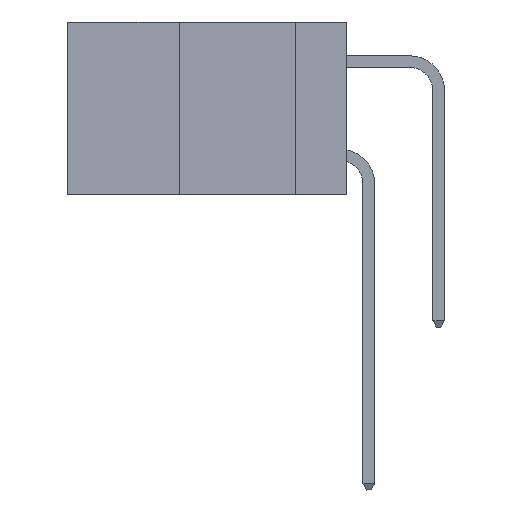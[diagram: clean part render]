
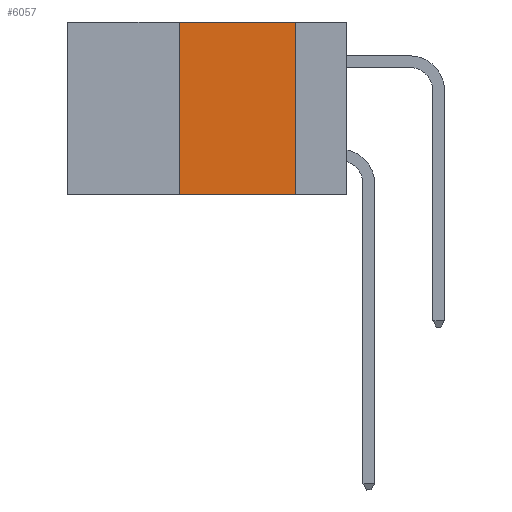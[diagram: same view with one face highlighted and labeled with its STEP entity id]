
A CAD part, left-side view. The second image highlights one B-rep face of the part: STEP entity #6057.
In plain terms, the highlighted planar face has unit normal (-1, 0, 0).
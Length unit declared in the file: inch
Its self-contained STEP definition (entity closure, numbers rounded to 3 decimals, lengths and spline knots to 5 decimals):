
#1659 = CARTESIAN_POINT ( 'NONE',  ( 0., 0.36, 0. ) ) ;
#2064 = AXIS2_PLACEMENT_3D ( 'NONE', #19146, #19528, #15060 ) ;
#2625 = VECTOR ( 'NONE', #18757, 39.37008 ) ;
#2629 = EDGE_CURVE ( 'NONE', #13762, #18556, #5952, .T. ) ;
#4824 = VECTOR ( 'NONE', #17352, 39.37008 ) ;
#4913 = CARTESIAN_POINT ( 'NONE',  ( 0., 0.36, -0.37 ) ) ;
#5952 = LINE ( 'NONE', #14203, #7526 ) ;
#6057 = ADVANCED_FACE ( 'NONE', ( #25244 ), #11332, .F. ) ;
#6169 = LINE ( 'NONE', #12888, #2625 ) ;
#7526 = VECTOR ( 'NONE', #21658, 39.37008 ) ;
#8325 = VERTEX_POINT ( 'NONE', #21366 ) ;
#9837 = EDGE_CURVE ( 'NONE', #8325, #16866, #6169, .T. ) ;
#10703 = CARTESIAN_POINT ( 'NONE',  ( 0., 0.11, 0. ) ) ;
#11332 = PLANE ( 'NONE',  #2064 ) ;
#12888 = CARTESIAN_POINT ( 'NONE',  ( 0., 0.6, 0. ) ) ;
#13762 = VERTEX_POINT ( 'NONE', #4913 ) ;
#14203 = CARTESIAN_POINT ( 'NONE',  ( 0., 0.6, -0.37 ) ) ;
#14489 = EDGE_LOOP ( 'NONE', ( #24083, #22445, #15694, #23614 ) ) ;
#14722 = DIRECTION ( 'NONE',  ( 0., 0., -1. ) ) ;
#15060 = DIRECTION ( 'NONE',  ( 0., 0., -1. ) ) ;
#15318 = LINE ( 'NONE', #1659, #4824 ) ;
#15694 = ORIENTED_EDGE ( 'NONE', *, *, #16026, .F. ) ;
#16026 = EDGE_CURVE ( 'NONE', #13762, #8325, #15318, .T. ) ;
#16866 = VERTEX_POINT ( 'NONE', #10703 ) ;
#17352 = DIRECTION ( 'NONE',  ( 0., 0., 1. ) ) ;
#18556 = VERTEX_POINT ( 'NONE', #21146 ) ;
#18757 = DIRECTION ( 'NONE',  ( 0., -1., 0. ) ) ;
#19146 = CARTESIAN_POINT ( 'NONE',  ( 0., 0.6, 0. ) ) ;
#19279 = EDGE_CURVE ( 'NONE', #16866, #18556, #20367, .T. ) ;
#19528 = DIRECTION ( 'NONE',  ( 1., 0., 0. ) ) ;
#20367 = LINE ( 'NONE', #24010, #22167 ) ;
#21146 = CARTESIAN_POINT ( 'NONE',  ( 0., 0.11, -0.37 ) ) ;
#21366 = CARTESIAN_POINT ( 'NONE',  ( 0., 0.36, 0. ) ) ;
#21658 = DIRECTION ( 'NONE',  ( 0., -1., 0. ) ) ;
#22167 = VECTOR ( 'NONE', #14722, 39.37008 ) ;
#22445 = ORIENTED_EDGE ( 'NONE', *, *, #9837, .F. ) ;
#23614 = ORIENTED_EDGE ( 'NONE', *, *, #2629, .T. ) ;
#24010 = CARTESIAN_POINT ( 'NONE',  ( 0., 0.11, 0. ) ) ;
#24083 = ORIENTED_EDGE ( 'NONE', *, *, #19279, .F. ) ;
#25244 = FACE_OUTER_BOUND ( 'NONE', #14489, .T. ) ;
